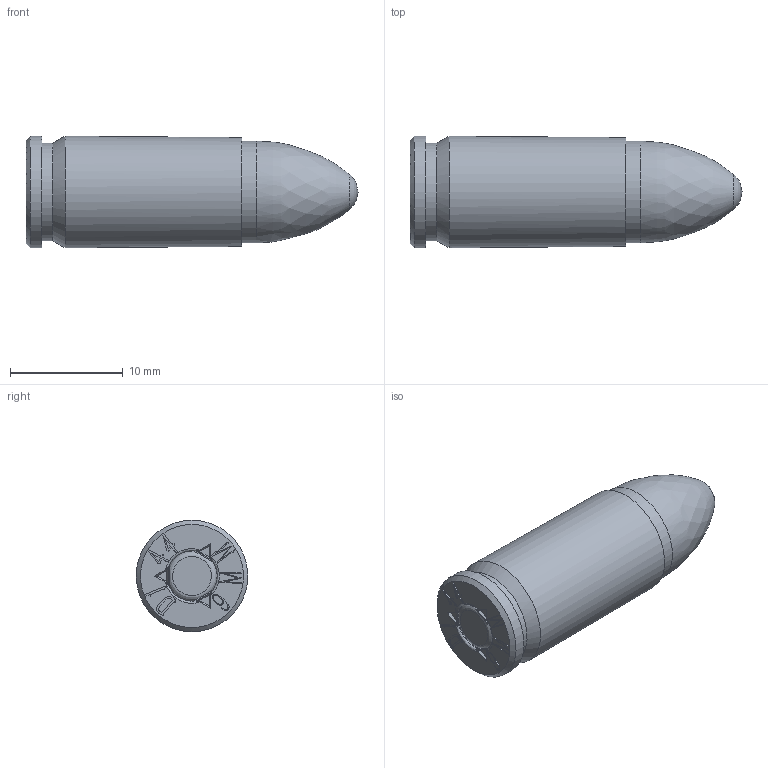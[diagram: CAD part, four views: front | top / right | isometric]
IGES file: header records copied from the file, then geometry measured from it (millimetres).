
Global section: file name: 9mm; native system: Autodesk Inventor 2019; preprocessor: unknown; author: user; date: 20200927.184102; units: millimetre
Bounding box: 29.4 x 9.87 x 9.88 mm (x, y, z)
Volume: 1224.4 mm3; surface area: 1698.3 mm2
Topology: 4 solids, 4 shells, 225 faces, 612 edges, 412 vertices
Faces by surface type: bspline 225
